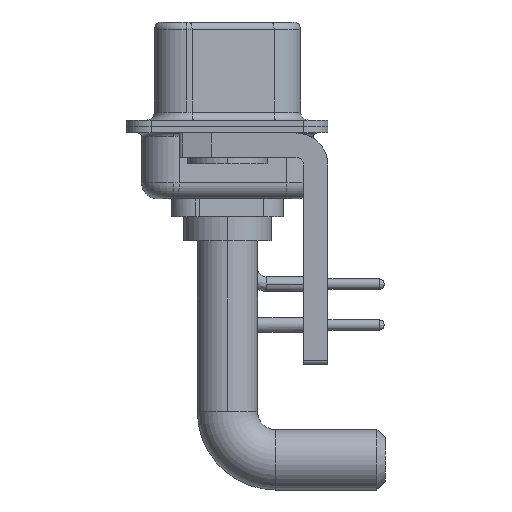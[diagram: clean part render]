
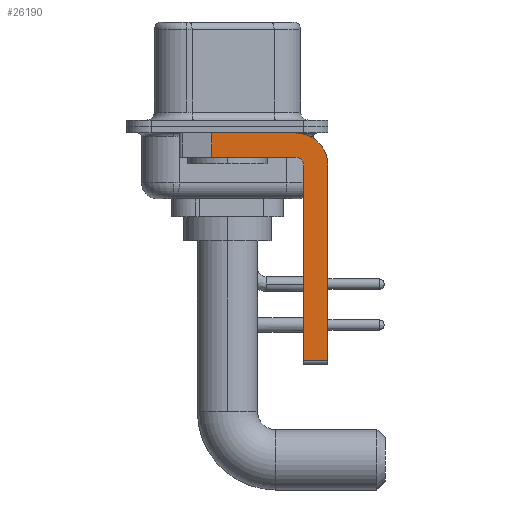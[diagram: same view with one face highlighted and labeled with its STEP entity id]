
A CAD part, left-side view. The second image highlights one B-rep face of the part: STEP entity #26190.
In plain terms, the highlighted planar face has unit normal (-1, 0, 0).
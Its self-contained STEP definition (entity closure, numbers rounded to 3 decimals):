
#1276 = VERTEX_POINT ( 'NONE', #7666 ) ;
#1699 = EDGE_CURVE ( 'NONE', #11250, #11892, #14116, .T. ) ;
#2130 = EDGE_CURVE ( 'NONE', #22154, #12054, #18344, .T. ) ;
#2254 = ORIENTED_EDGE ( 'NONE', *, *, #21391, .F. ) ;
#2571 = VERTEX_POINT ( 'NONE', #16748 ) ;
#3606 = ORIENTED_EDGE ( 'NONE', *, *, #8482, .F. ) ;
#4536 = CIRCLE ( 'NONE', #27223, 0.5 ) ;
#6217 = EDGE_CURVE ( 'NONE', #23721, #11548, #4536, .T. ) ;
#6965 = DIRECTION ( 'NONE',  ( -1., 0., 0. ) ) ;
#7199 = CARTESIAN_POINT ( 'NONE',  ( -2.9, -4.25, -2.4 ) ) ;
#7369 = CARTESIAN_POINT ( 'NONE',  ( -2.9, 0.978, -0.4 ) ) ;
#7666 = CARTESIAN_POINT ( 'NONE',  ( -2.9, -4.75, -14.55 ) ) ;
#7788 = VECTOR ( 'NONE', #12155, 1000. ) ;
#8474 = AXIS2_PLACEMENT_3D ( 'NONE', #12548, #21053, #10456 ) ;
#8482 = EDGE_CURVE ( 'NONE', #1276, #23721, #9314, .T. ) ;
#8504 = EDGE_LOOP ( 'NONE', ( #21343, #21028, #2254, #17174, #3606, #13602, #24872, #20954 ) ) ;
#8730 = CARTESIAN_POINT ( 'NONE',  ( -2.9, -4.75, -2.4 ) ) ;
#8959 = EDGE_CURVE ( 'NONE', #11250, #2571, #9939, .T. ) ;
#9314 = LINE ( 'NONE', #22407, #16637 ) ;
#9665 = CARTESIAN_POINT ( 'NONE',  ( -2.9, -4.25, -14.55 ) ) ;
#9939 = LINE ( 'NONE', #11885, #16226 ) ;
#9951 = CARTESIAN_POINT ( 'NONE',  ( -2.9, -6.25, -2.4 ) ) ;
#10078 = EDGE_CURVE ( 'NONE', #1276, #12054, #13441, .T. ) ;
#10456 = DIRECTION ( 'NONE',  ( 0., 0., -1. ) ) ;
#11250 = VERTEX_POINT ( 'NONE', #7369 ) ;
#11515 = DIRECTION ( 'NONE',  ( 0., 0., -1. ) ) ;
#11548 = VERTEX_POINT ( 'NONE', #15541 ) ;
#11885 = CARTESIAN_POINT ( 'NONE',  ( -2.9, 0.978, -1.9 ) ) ;
#11892 = VERTEX_POINT ( 'NONE', #13148 ) ;
#12054 = VERTEX_POINT ( 'NONE', #13422 ) ;
#12155 = DIRECTION ( 'NONE',  ( 0., -1., 0. ) ) ;
#12296 = DIRECTION ( 'NONE',  ( 0., 0., -1. ) ) ;
#12548 = CARTESIAN_POINT ( 'NONE',  ( -2.9, -4.25, -2.4 ) ) ;
#13148 = CARTESIAN_POINT ( 'NONE',  ( -2.9, -4.25, -0.4 ) ) ;
#13422 = CARTESIAN_POINT ( 'NONE',  ( -2.9, -6.25, -14.55 ) ) ;
#13441 = LINE ( 'NONE', #9665, #19444 ) ;
#13602 = ORIENTED_EDGE ( 'NONE', *, *, #10078, .T. ) ;
#13995 = DIRECTION ( 'NONE',  ( 0., -1., 0. ) ) ;
#14041 = DIRECTION ( 'NONE',  ( 0., 0., 1. ) ) ;
#14116 = LINE ( 'NONE', #22618, #7788 ) ;
#14759 = EDGE_CURVE ( 'NONE', #11892, #22154, #26709, .T. ) ;
#15541 = CARTESIAN_POINT ( 'NONE',  ( -2.9, -4.25, -1.9 ) ) ;
#16226 = VECTOR ( 'NONE', #12296, 1000. ) ;
#16637 = VECTOR ( 'NONE', #14041, 1000. ) ;
#16667 = DIRECTION ( 'NONE',  ( 0., 0., -1. ) ) ;
#16748 = CARTESIAN_POINT ( 'NONE',  ( -2.9, 0.978, -1.9 ) ) ;
#17174 = ORIENTED_EDGE ( 'NONE', *, *, #6217, .F. ) ;
#17356 = AXIS2_PLACEMENT_3D ( 'NONE', #7199, #22112, #11515 ) ;
#17547 = LINE ( 'NONE', #20053, #20980 ) ;
#17785 = PLANE ( 'NONE',  #17356 ) ;
#18344 = LINE ( 'NONE', #27274, #27372 ) ;
#19444 = VECTOR ( 'NONE', #13995, 1000. ) ;
#19878 = FACE_OUTER_BOUND ( 'NONE', #8504, .T. ) ;
#19911 = DIRECTION ( 'NONE',  ( 0., 1., 0. ) ) ;
#20053 = CARTESIAN_POINT ( 'NONE',  ( -2.9, -4.25, -1.9 ) ) ;
#20954 = ORIENTED_EDGE ( 'NONE', *, *, #14759, .F. ) ;
#20980 = VECTOR ( 'NONE', #19911, 1000. ) ;
#21028 = ORIENTED_EDGE ( 'NONE', *, *, #8959, .T. ) ;
#21053 = DIRECTION ( 'NONE',  ( 1., 0., 0. ) ) ;
#21343 = ORIENTED_EDGE ( 'NONE', *, *, #1699, .F. ) ;
#21391 = EDGE_CURVE ( 'NONE', #11548, #2571, #17547, .T. ) ;
#22112 = DIRECTION ( 'NONE',  ( 1., 0., 0. ) ) ;
#22154 = VERTEX_POINT ( 'NONE', #9951 ) ;
#22407 = CARTESIAN_POINT ( 'NONE',  ( -2.9, -4.75, -14.8 ) ) ;
#22618 = CARTESIAN_POINT ( 'NONE',  ( -2.9, 3., -0.4 ) ) ;
#23721 = VERTEX_POINT ( 'NONE', #8730 ) ;
#23973 = DIRECTION ( 'NONE',  ( 0., 0., 1. ) ) ;
#24872 = ORIENTED_EDGE ( 'NONE', *, *, #2130, .F. ) ;
#26067 = CARTESIAN_POINT ( 'NONE',  ( -2.9, -4.25, -2.4 ) ) ;
#26190 = ADVANCED_FACE ( 'NONE', ( #19878 ), #17785, .F. ) ;
#26709 = CIRCLE ( 'NONE', #8474, 2. ) ;
#27223 = AXIS2_PLACEMENT_3D ( 'NONE', #26067, #6965, #23973 ) ;
#27274 = CARTESIAN_POINT ( 'NONE',  ( -2.9, -6.25, -2.4 ) ) ;
#27372 = VECTOR ( 'NONE', #16667, 1000. ) ;
